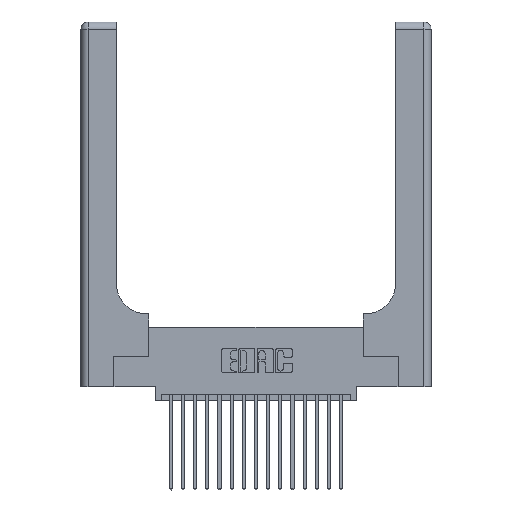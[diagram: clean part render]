
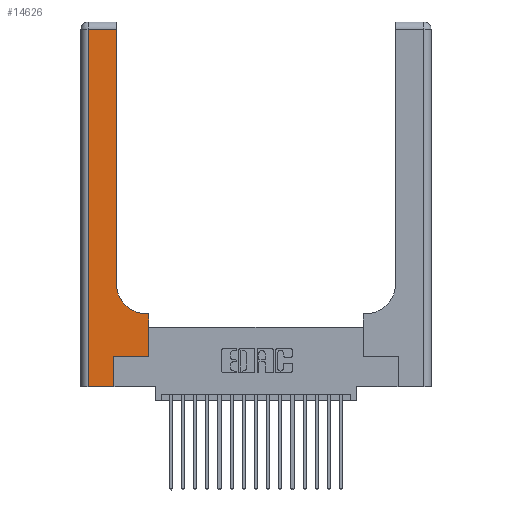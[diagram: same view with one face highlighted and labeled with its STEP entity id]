
A CAD part, top view. The second image highlights one B-rep face of the part: STEP entity #14626.
In plain terms, the highlighted planar face has unit normal (0, 0, 1).
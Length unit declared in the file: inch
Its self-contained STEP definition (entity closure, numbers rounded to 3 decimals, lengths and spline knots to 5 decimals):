
#191 = VECTOR ( 'NONE', #10127, 39.37008 ) ;
#977 = ORIENTED_EDGE ( 'NONE', *, *, #5704, .T. ) ;
#1123 = PLANE ( 'NONE',  #11848 ) ;
#1365 = DIRECTION ( 'NONE',  ( 0., 1., 0. ) ) ;
#1903 = CARTESIAN_POINT ( 'NONE',  ( 0.269, 0.25, 0.37 ) ) ;
#2249 = LINE ( 'NONE', #13655, #20603 ) ;
#2753 = DIRECTION ( 'NONE',  ( 1., 0., 0. ) ) ;
#3076 = FACE_OUTER_BOUND ( 'NONE', #7874, .T. ) ;
#3727 = CARTESIAN_POINT ( 'NONE',  ( 0., 0., 0.37 ) ) ;
#3737 = AXIS2_PLACEMENT_3D ( 'NONE', #4445, #18995, #2753 ) ;
#4124 = CARTESIAN_POINT ( 'NONE',  ( 0.269, 0., 0.37 ) ) ;
#4313 = VECTOR ( 'NONE', #14739, 39.37008 ) ;
#4442 = DIRECTION ( 'NONE',  ( 0., 0., -1. ) ) ;
#4445 = CARTESIAN_POINT ( 'NONE',  ( 0.5415, 0.85, 0.37 ) ) ;
#4972 = ORIENTED_EDGE ( 'NONE', *, *, #16080, .T. ) ;
#5033 = VERTEX_POINT ( 'NONE', #18006 ) ;
#5258 = EDGE_CURVE ( 'NONE', #12556, #11150, #14852, .T. ) ;
#5407 = LINE ( 'NONE', #11707, #191 ) ;
#5704 = EDGE_CURVE ( 'NONE', #11150, #9693, #14210, .T. ) ;
#6260 = VECTOR ( 'NONE', #17152, 39.37008 ) ;
#6299 = VECTOR ( 'NONE', #6973, 39.37008 ) ;
#6339 = CARTESIAN_POINT ( 'NONE',  ( 0.5585, 0.25, 0.37 ) ) ;
#6635 = VERTEX_POINT ( 'NONE', #10306 ) ;
#6973 = DIRECTION ( 'NONE',  ( 1., 0., 0. ) ) ;
#7151 = DIRECTION ( 'NONE',  ( 0., 1., 0. ) ) ;
#7334 = VECTOR ( 'NONE', #18140, 39.37008 ) ;
#7511 = ORIENTED_EDGE ( 'NONE', *, *, #7724, .T. ) ;
#7641 = VERTEX_POINT ( 'NONE', #10399 ) ;
#7724 = EDGE_CURVE ( 'NONE', #18900, #8548, #19859, .T. ) ;
#7874 = EDGE_LOOP ( 'NONE', ( #4972, #14680, #9791, #11161, #977, #8902, #7511, #13689, #10825 ) ) ;
#8075 = LINE ( 'NONE', #16522, #7334 ) ;
#8548 = VERTEX_POINT ( 'NONE', #13877 ) ;
#8902 = ORIENTED_EDGE ( 'NONE', *, *, #9575, .T. ) ;
#9171 = DIRECTION ( 'NONE',  ( -1., 0., 0. ) ) ;
#9575 = EDGE_CURVE ( 'NONE', #9693, #18900, #19087, .T. ) ;
#9693 = VERTEX_POINT ( 'NONE', #18210 ) ;
#9791 = ORIENTED_EDGE ( 'NONE', *, *, #15536, .T. ) ;
#9816 = VECTOR ( 'NONE', #1365, 39.37008 ) ;
#9889 = CARTESIAN_POINT ( 'NONE',  ( 0.06, 3., 0.37 ) ) ;
#10127 = DIRECTION ( 'NONE',  ( -1., 0., 0. ) ) ;
#10273 = CARTESIAN_POINT ( 'NONE',  ( 0.06, 0., 0.37 ) ) ;
#10306 = CARTESIAN_POINT ( 'NONE',  ( 0.2915, 0.85, 0.37 ) ) ;
#10380 = CARTESIAN_POINT ( 'NONE',  ( 0.2915, 2.94, 0.37 ) ) ;
#10399 = CARTESIAN_POINT ( 'NONE',  ( 0.5415, 0.6, 0.37 ) ) ;
#10825 = ORIENTED_EDGE ( 'NONE', *, *, #16286, .T. ) ;
#11150 = VERTEX_POINT ( 'NONE', #18885 ) ;
#11161 = ORIENTED_EDGE ( 'NONE', *, *, #5258, .T. ) ;
#11276 = EDGE_CURVE ( 'NONE', #8548, #7641, #5407, .T. ) ;
#11707 = CARTESIAN_POINT ( 'NONE',  ( 0.2915, 0.6, 0.37 ) ) ;
#11848 = AXIS2_PLACEMENT_3D ( 'NONE', #20309, #4442, #9171 ) ;
#12556 = VERTEX_POINT ( 'NONE', #10273 ) ;
#13109 = LINE ( 'NONE', #9889, #4313 ) ;
#13655 = CARTESIAN_POINT ( 'NONE',  ( 0., 2.94, 0.37 ) ) ;
#13689 = ORIENTED_EDGE ( 'NONE', *, *, #11276, .T. ) ;
#13877 = CARTESIAN_POINT ( 'NONE',  ( 0.5585, 0.6, 0.37 ) ) ;
#14210 = LINE ( 'NONE', #4124, #17466 ) ;
#14626 = ADVANCED_FACE ( 'NONE', ( #3076 ), #1123, .F. ) ;
#14680 = ORIENTED_EDGE ( 'NONE', *, *, #17251, .T. ) ;
#14739 = DIRECTION ( 'NONE',  ( 0., -1., 0. ) ) ;
#14852 = LINE ( 'NONE', #3727, #6299 ) ;
#15116 = CIRCLE ( 'NONE', #3737, 0.25 ) ;
#15280 = DIRECTION ( 'NONE',  ( -1., 0., 0. ) ) ;
#15536 = EDGE_CURVE ( 'NONE', #5033, #12556, #13109, .T. ) ;
#16080 = EDGE_CURVE ( 'NONE', #6635, #18845, #8075, .T. ) ;
#16286 = EDGE_CURVE ( 'NONE', #7641, #6635, #15116, .T. ) ;
#16522 = CARTESIAN_POINT ( 'NONE',  ( 0.2915, 3., 0.37 ) ) ;
#17152 = DIRECTION ( 'NONE',  ( 1., 0., 0. ) ) ;
#17251 = EDGE_CURVE ( 'NONE', #18845, #5033, #2249, .T. ) ;
#17466 = VECTOR ( 'NONE', #7151, 39.37008 ) ;
#18006 = CARTESIAN_POINT ( 'NONE',  ( 0.06, 2.94, 0.37 ) ) ;
#18140 = DIRECTION ( 'NONE',  ( 0., 1., 0. ) ) ;
#18210 = CARTESIAN_POINT ( 'NONE',  ( 0.269, 0.25, 0.37 ) ) ;
#18845 = VERTEX_POINT ( 'NONE', #10380 ) ;
#18885 = CARTESIAN_POINT ( 'NONE',  ( 0.269, 0., 0.37 ) ) ;
#18900 = VERTEX_POINT ( 'NONE', #6339 ) ;
#18995 = DIRECTION ( 'NONE',  ( 0., 0., -1. ) ) ;
#19087 = LINE ( 'NONE', #1903, #6260 ) ;
#19118 = CARTESIAN_POINT ( 'NONE',  ( 0.5585, 0.25, 0.37 ) ) ;
#19859 = LINE ( 'NONE', #19118, #9816 ) ;
#20309 = CARTESIAN_POINT ( 'NONE',  ( 0., 3., 0.37 ) ) ;
#20603 = VECTOR ( 'NONE', #15280, 39.37008 ) ;
